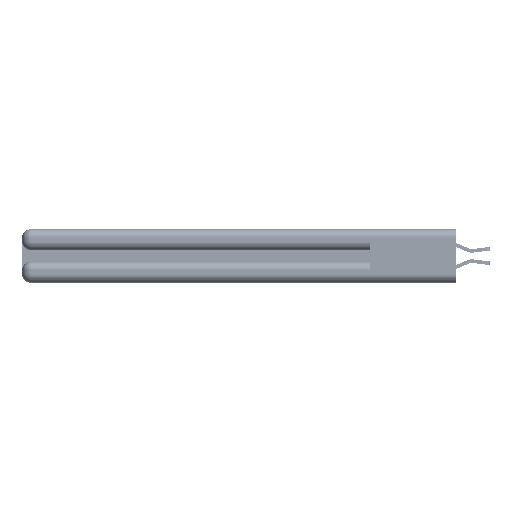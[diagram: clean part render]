
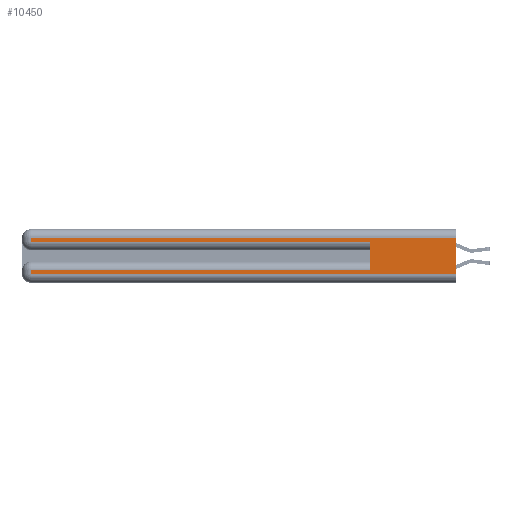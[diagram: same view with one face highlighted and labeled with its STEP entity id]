
A CAD part, left-side view. The second image highlights one B-rep face of the part: STEP entity #10450.
In plain terms, the highlighted planar face has unit normal (-1, 0, 0).
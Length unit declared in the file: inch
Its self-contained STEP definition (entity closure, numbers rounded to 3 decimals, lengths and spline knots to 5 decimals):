
#51 = CARTESIAN_POINT ( 'NONE',  ( 0., 0., 0.06 ) ) ;
#331 = ORIENTED_EDGE ( 'NONE', *, *, #15835, .T. ) ;
#1131 = LINE ( 'NONE', #51, #26193 ) ;
#2188 = ORIENTED_EDGE ( 'NONE', *, *, #41886, .T. ) ;
#3107 = ORIENTED_EDGE ( 'NONE', *, *, #10534, .T. ) ;
#3608 = DIRECTION ( 'NONE',  ( 0., 1., 0. ) ) ;
#5602 = EDGE_CURVE ( 'NONE', #38195, #32857, #34593, .T. ) ;
#7541 = AXIS2_PLACEMENT_3D ( 'NONE', #13005, #9551, #22863 ) ;
#7812 = CARTESIAN_POINT ( 'NONE',  ( 0., 0., 0.31 ) ) ;
#7890 = VERTEX_POINT ( 'NONE', #7946 ) ;
#7946 = CARTESIAN_POINT ( 'NONE',  ( 0., 2.94, 0.06 ) ) ;
#9063 = VERTEX_POINT ( 'NONE', #41785 ) ;
#9429 = VERTEX_POINT ( 'NONE', #36660 ) ;
#9551 = DIRECTION ( 'NONE',  ( 1., 0., 0. ) ) ;
#9590 = DIRECTION ( 'NONE',  ( 0., 0., -1. ) ) ;
#9654 = DIRECTION ( 'NONE',  ( 0., 0., -1. ) ) ;
#9769 = DIRECTION ( 'NONE',  ( 0., 0., -1. ) ) ;
#9916 = ORIENTED_EDGE ( 'NONE', *, *, #38507, .F. ) ;
#10050 = EDGE_CURVE ( 'NONE', #9429, #29606, #34762, .T. ) ;
#10450 = ADVANCED_FACE ( 'NONE', ( #39290 ), #19706, .F. ) ;
#10534 = EDGE_CURVE ( 'NONE', #32857, #9063, #15759, .T. ) ;
#10999 = VECTOR ( 'NONE', #9654, 39.37008 ) ;
#11207 = DIRECTION ( 'NONE',  ( 0., 0., 1. ) ) ;
#13005 = CARTESIAN_POINT ( 'NONE',  ( 0., 0., 0.37 ) ) ;
#13140 = CARTESIAN_POINT ( 'NONE',  ( 0., 2.94, 0.085 ) ) ;
#13211 = VECTOR ( 'NONE', #36149, 39.37008 ) ;
#14723 = LINE ( 'NONE', #34407, #38722 ) ;
#15759 = LINE ( 'NONE', #33428, #13211 ) ;
#15835 = EDGE_CURVE ( 'NONE', #29606, #7890, #21252, .T. ) ;
#17088 = ORIENTED_EDGE ( 'NONE', *, *, #33317, .F. ) ;
#17154 = VECTOR ( 'NONE', #9590, 39.37008 ) ;
#17996 = ORIENTED_EDGE ( 'NONE', *, *, #10050, .T. ) ;
#19706 = PLANE ( 'NONE',  #7541 ) ;
#20779 = ORIENTED_EDGE ( 'NONE', *, *, #5602, .T. ) ;
#21252 = LINE ( 'NONE', #29247, #10999 ) ;
#22863 = DIRECTION ( 'NONE',  ( 0., 0., -1. ) ) ;
#23567 = LINE ( 'NONE', #33238, #38422 ) ;
#23982 = VECTOR ( 'NONE', #39619, 39.37008 ) ;
#25857 = LINE ( 'NONE', #39961, #33078 ) ;
#26193 = VECTOR ( 'NONE', #36231, 39.37008 ) ;
#27786 = CARTESIAN_POINT ( 'NONE',  ( 0., 2.94, 0.31 ) ) ;
#28707 = ORIENTED_EDGE ( 'NONE', *, *, #36123, .T. ) ;
#29247 = CARTESIAN_POINT ( 'NONE',  ( 0., 2.94, 0.37 ) ) ;
#29321 = CARTESIAN_POINT ( 'NONE',  ( 0., 0., 0.085 ) ) ;
#29606 = VERTEX_POINT ( 'NONE', #13140 ) ;
#30014 = VERTEX_POINT ( 'NONE', #7812 ) ;
#32857 = VERTEX_POINT ( 'NONE', #42028 ) ;
#33078 = VECTOR ( 'NONE', #3608, 39.37008 ) ;
#33238 = CARTESIAN_POINT ( 'NONE',  ( 0., 0., 0.37 ) ) ;
#33317 = EDGE_CURVE ( 'NONE', #9429, #9063, #14723, .T. ) ;
#33428 = CARTESIAN_POINT ( 'NONE',  ( 0., 0., 0.285 ) ) ;
#34407 = CARTESIAN_POINT ( 'NONE',  ( 0., 0.6, 0.145 ) ) ;
#34593 = LINE ( 'NONE', #42088, #17154 ) ;
#34607 = VERTEX_POINT ( 'NONE', #35952 ) ;
#34762 = LINE ( 'NONE', #29321, #23982 ) ;
#35952 = CARTESIAN_POINT ( 'NONE',  ( 0., 0., 0.06 ) ) ;
#36123 = EDGE_CURVE ( 'NONE', #7890, #34607, #1131, .T. ) ;
#36149 = DIRECTION ( 'NONE',  ( 0., -1., 0. ) ) ;
#36231 = DIRECTION ( 'NONE',  ( 0., -1., 0. ) ) ;
#36660 = CARTESIAN_POINT ( 'NONE',  ( 0., 0.6, 0.085 ) ) ;
#38195 = VERTEX_POINT ( 'NONE', #27786 ) ;
#38422 = VECTOR ( 'NONE', #9769, 39.37008 ) ;
#38507 = EDGE_CURVE ( 'NONE', #30014, #34607, #23567, .T. ) ;
#38722 = VECTOR ( 'NONE', #11207, 39.37008 ) ;
#39290 = FACE_OUTER_BOUND ( 'NONE', #42254, .T. ) ;
#39619 = DIRECTION ( 'NONE',  ( 0., 1., 0. ) ) ;
#39961 = CARTESIAN_POINT ( 'NONE',  ( 0., 0., 0.31 ) ) ;
#41785 = CARTESIAN_POINT ( 'NONE',  ( 0., 0.6, 0.285 ) ) ;
#41886 = EDGE_CURVE ( 'NONE', #30014, #38195, #25857, .T. ) ;
#42028 = CARTESIAN_POINT ( 'NONE',  ( 0., 2.94, 0.285 ) ) ;
#42088 = CARTESIAN_POINT ( 'NONE',  ( 0., 2.94, 0.37 ) ) ;
#42254 = EDGE_LOOP ( 'NONE', ( #9916, #2188, #20779, #3107, #17088, #17996, #331, #28707 ) ) ;
